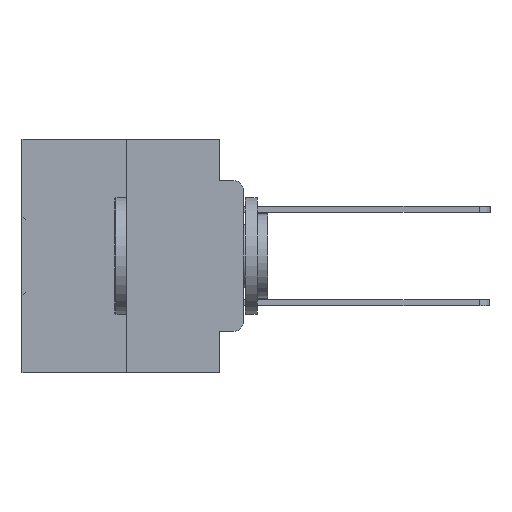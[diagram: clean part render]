
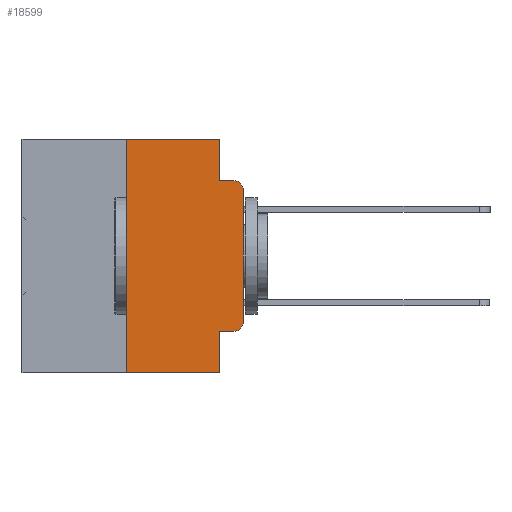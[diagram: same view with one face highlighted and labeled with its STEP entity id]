
A CAD part, left-side view. The second image highlights one B-rep face of the part: STEP entity #18599.
In plain terms, the highlighted planar face has unit normal (-1, 0, 0).
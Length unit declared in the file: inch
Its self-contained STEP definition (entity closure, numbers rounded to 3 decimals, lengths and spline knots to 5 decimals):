
#273 = EDGE_CURVE ( 'NONE', #27498, #20293, #25166, .T. ) ;
#455 = CARTESIAN_POINT ( 'NONE',  ( 0., 0.051, -0.4115 ) ) ;
#937 = EDGE_CURVE ( 'NONE', #8486, #6307, #8608, .T. ) ;
#1567 = CARTESIAN_POINT ( 'NONE',  ( 0., 0.473, -0.5 ) ) ;
#1793 = LINE ( 'NONE', #1567, #8172 ) ;
#2423 = ORIENTED_EDGE ( 'NONE', *, *, #28190, .F. ) ;
#2617 = LINE ( 'NONE', #4437, #9010 ) ;
#2778 = LINE ( 'NONE', #3704, #16302 ) ;
#3053 = LINE ( 'NONE', #3354, #16566 ) ;
#3212 = AXIS2_PLACEMENT_3D ( 'NONE', #17896, #18052, #18020 ) ;
#3354 = CARTESIAN_POINT ( 'NONE',  ( 0., 0.051, 0. ) ) ;
#3704 = CARTESIAN_POINT ( 'NONE',  ( 0., 0.051, -0.4115 ) ) ;
#3925 = EDGE_CURVE ( 'NONE', #6307, #27498, #13472, .T. ) ;
#4146 = ORIENTED_EDGE ( 'NONE', *, *, #16625, .F. ) ;
#4341 = PLANE ( 'NONE',  #25967 ) ;
#4437 = CARTESIAN_POINT ( 'NONE',  ( 0., 0.051, -0.0885 ) ) ;
#5374 = EDGE_LOOP ( 'NONE', ( #24421, #21451, #23159, #2423, #4146, #6691, #22752, #10118, #17217, #12661 ) ) ;
#5540 = CARTESIAN_POINT ( 'NONE',  ( 0., 0.051, 0. ) ) ;
#5579 = CARTESIAN_POINT ( 'NONE',  ( 0., 0.25, 0. ) ) ;
#6221 = CARTESIAN_POINT ( 'NONE',  ( 0., 0.051, 0. ) ) ;
#6307 = VERTEX_POINT ( 'NONE', #11860 ) ;
#6691 = ORIENTED_EDGE ( 'NONE', *, *, #22711, .F. ) ;
#8172 = VECTOR ( 'NONE', #31368, 39.37008 ) ;
#8448 = CARTESIAN_POINT ( 'NONE',  ( 0., 0.25, 0. ) ) ;
#8486 = VERTEX_POINT ( 'NONE', #18043 ) ;
#8608 = CIRCLE ( 'NONE', #3212, 0.02 ) ;
#9010 = VECTOR ( 'NONE', #9783, 39.37008 ) ;
#9176 = DIRECTION ( 'NONE',  ( 0., -1., 0. ) ) ;
#9739 = VERTEX_POINT ( 'NONE', #10398 ) ;
#9783 = DIRECTION ( 'NONE',  ( 0., -1., 0. ) ) ;
#10081 = EDGE_CURVE ( 'NONE', #24656, #8486, #2778, .T. ) ;
#10118 = ORIENTED_EDGE ( 'NONE', *, *, #19039, .F. ) ;
#10398 = CARTESIAN_POINT ( 'NONE',  ( 0., 0.051, -0.5 ) ) ;
#11860 = CARTESIAN_POINT ( 'NONE',  ( 0., 0., -0.3915 ) ) ;
#12543 = DIRECTION ( 'NONE',  ( 1., 0., 0. ) ) ;
#12633 = DIRECTION ( 'NONE',  ( 0., -1., 0. ) ) ;
#12651 = VECTOR ( 'NONE', #21254, 39.37008 ) ;
#12661 = ORIENTED_EDGE ( 'NONE', *, *, #937, .T. ) ;
#13194 = LINE ( 'NONE', #6221, #34619 ) ;
#13414 = LINE ( 'NONE', #5579, #19690 ) ;
#13472 = LINE ( 'NONE', #34051, #12651 ) ;
#14594 = EDGE_CURVE ( 'NONE', #16570, #9739, #1793, .T. ) ;
#15239 = LINE ( 'NONE', #34122, #27983 ) ;
#15573 = CARTESIAN_POINT ( 'NONE',  ( 0., 0.051, -0.0885 ) ) ;
#16302 = VECTOR ( 'NONE', #9176, 39.37008 ) ;
#16566 = VECTOR ( 'NONE', #19506, 39.37008 ) ;
#16570 = VERTEX_POINT ( 'NONE', #33785 ) ;
#16610 = CARTESIAN_POINT ( 'NONE',  ( 0., 0., -0.1085 ) ) ;
#16625 = EDGE_CURVE ( 'NONE', #26263, #25179, #15239, .T. ) ;
#17217 = ORIENTED_EDGE ( 'NONE', *, *, #10081, .T. ) ;
#17896 = CARTESIAN_POINT ( 'NONE',  ( 0., 0.02, -0.3915 ) ) ;
#18020 = DIRECTION ( 'NONE',  ( 0., 0., -1. ) ) ;
#18043 = CARTESIAN_POINT ( 'NONE',  ( 0., 0.02, -0.4115 ) ) ;
#18052 = DIRECTION ( 'NONE',  ( -1., 0., 0. ) ) ;
#18599 = ADVANCED_FACE ( 'NONE', ( #22966 ), #4341, .F. ) ;
#19039 = EDGE_CURVE ( 'NONE', #24656, #9739, #3053, .T. ) ;
#19506 = DIRECTION ( 'NONE',  ( 0., 0., -1. ) ) ;
#19635 = DIRECTION ( 'NONE',  ( 0., 0., -1. ) ) ;
#19690 = VECTOR ( 'NONE', #21732, 39.37008 ) ;
#19890 = VERTEX_POINT ( 'NONE', #15573 ) ;
#20034 = CARTESIAN_POINT ( 'NONE',  ( 0., 0.02, -0.0885 ) ) ;
#20293 = VERTEX_POINT ( 'NONE', #20034 ) ;
#21254 = DIRECTION ( 'NONE',  ( 0., 0., 1. ) ) ;
#21451 = ORIENTED_EDGE ( 'NONE', *, *, #273, .T. ) ;
#21524 = AXIS2_PLACEMENT_3D ( 'NONE', #24509, #29529, #25334 ) ;
#21732 = DIRECTION ( 'NONE',  ( 0., 0., 1. ) ) ;
#22711 = EDGE_CURVE ( 'NONE', #16570, #26263, #13414, .T. ) ;
#22752 = ORIENTED_EDGE ( 'NONE', *, *, #14594, .T. ) ;
#22966 = FACE_OUTER_BOUND ( 'NONE', #5374, .T. ) ;
#23159 = ORIENTED_EDGE ( 'NONE', *, *, #31746, .F. ) ;
#24421 = ORIENTED_EDGE ( 'NONE', *, *, #3925, .T. ) ;
#24509 = CARTESIAN_POINT ( 'NONE',  ( 0., 0.02, -0.1085 ) ) ;
#24656 = VERTEX_POINT ( 'NONE', #455 ) ;
#25166 = CIRCLE ( 'NONE', #21524, 0.02 ) ;
#25179 = VERTEX_POINT ( 'NONE', #5540 ) ;
#25334 = DIRECTION ( 'NONE',  ( 0., 0., -1. ) ) ;
#25967 = AXIS2_PLACEMENT_3D ( 'NONE', #25989, #12543, #31377 ) ;
#25989 = CARTESIAN_POINT ( 'NONE',  ( 0., 0.473, 0. ) ) ;
#26263 = VERTEX_POINT ( 'NONE', #8448 ) ;
#27498 = VERTEX_POINT ( 'NONE', #16610 ) ;
#27983 = VECTOR ( 'NONE', #12633, 39.37008 ) ;
#28190 = EDGE_CURVE ( 'NONE', #25179, #19890, #13194, .T. ) ;
#29529 = DIRECTION ( 'NONE',  ( -1., 0., 0. ) ) ;
#31368 = DIRECTION ( 'NONE',  ( 0., -1., 0. ) ) ;
#31377 = DIRECTION ( 'NONE',  ( 0., 0., -1. ) ) ;
#31746 = EDGE_CURVE ( 'NONE', #19890, #20293, #2617, .T. ) ;
#33785 = CARTESIAN_POINT ( 'NONE',  ( 0., 0.25, -0.5 ) ) ;
#34051 = CARTESIAN_POINT ( 'NONE',  ( 0., 0., 0. ) ) ;
#34122 = CARTESIAN_POINT ( 'NONE',  ( 0., 0.473, 0. ) ) ;
#34619 = VECTOR ( 'NONE', #19635, 39.37008 ) ;
